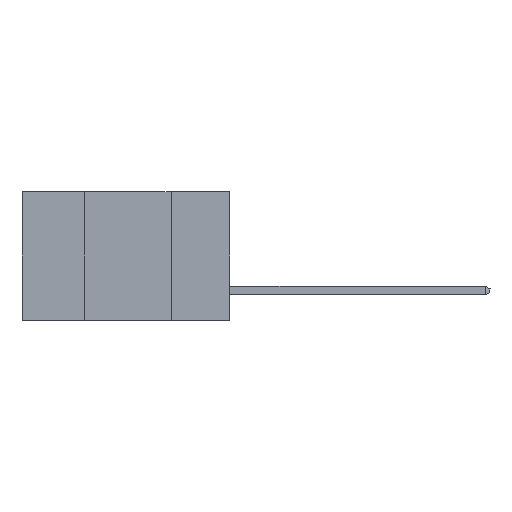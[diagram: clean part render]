
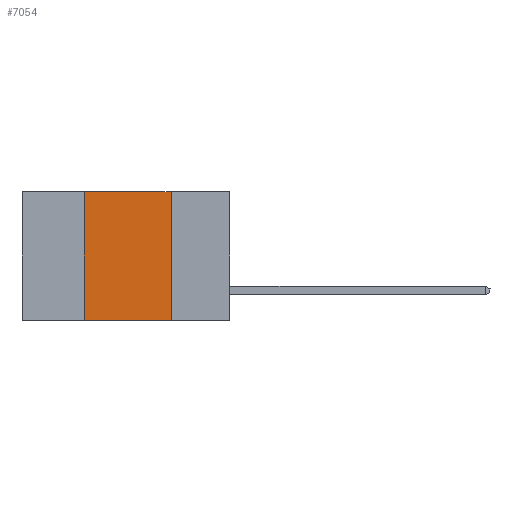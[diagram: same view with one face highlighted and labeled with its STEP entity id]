
A CAD part, left-side view. The second image highlights one B-rep face of the part: STEP entity #7054.
In plain terms, the highlighted planar face has unit normal (-1, 0, 0).
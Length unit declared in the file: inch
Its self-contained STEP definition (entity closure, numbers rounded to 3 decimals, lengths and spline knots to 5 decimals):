
#349 = CARTESIAN_POINT ( 'NONE',  ( 0., 0.6, 0. ) ) ;
#398 = VECTOR ( 'NONE', #7942, 39.37008 ) ;
#472 = CARTESIAN_POINT ( 'NONE',  ( 0., 0.17, 0. ) ) ;
#511 = CARTESIAN_POINT ( 'NONE',  ( 0., 0.42, 0. ) ) ;
#858 = VECTOR ( 'NONE', #1346, 39.37008 ) ;
#1288 = CARTESIAN_POINT ( 'NONE',  ( 0., 0.17, -0.37 ) ) ;
#1346 = DIRECTION ( 'NONE',  ( 0., -1., 0. ) ) ;
#2298 = CARTESIAN_POINT ( 'NONE',  ( 0., 0.6, -0.37 ) ) ;
#2916 = EDGE_CURVE ( 'NONE', #11354, #6321, #6227, .T. ) ;
#3241 = LINE ( 'NONE', #349, #7629 ) ;
#3718 = DIRECTION ( 'NONE',  ( 0., 0., -1. ) ) ;
#3831 = VECTOR ( 'NONE', #9701, 39.37008 ) ;
#4133 = LINE ( 'NONE', #8748, #398 ) ;
#4154 = EDGE_CURVE ( 'NONE', #11354, #4157, #5751, .T. ) ;
#4157 = VERTEX_POINT ( 'NONE', #511 ) ;
#5074 = EDGE_CURVE ( 'NONE', #4157, #11712, #3241, .T. ) ;
#5171 = ORIENTED_EDGE ( 'NONE', *, *, #12190, .F. ) ;
#5327 = FACE_OUTER_BOUND ( 'NONE', #8005, .T. ) ;
#5512 = DIRECTION ( 'NONE',  ( 1., 0., 0. ) ) ;
#5751 = LINE ( 'NONE', #5878, #3831 ) ;
#5878 = CARTESIAN_POINT ( 'NONE',  ( 0., 0.42, -0.37 ) ) ;
#6039 = DIRECTION ( 'NONE',  ( 0., -1., 0. ) ) ;
#6227 = LINE ( 'NONE', #2298, #858 ) ;
#6321 = VERTEX_POINT ( 'NONE', #1288 ) ;
#7054 = ADVANCED_FACE ( 'NONE', ( #5327 ), #10348, .F. ) ;
#7629 = VECTOR ( 'NONE', #6039, 39.37008 ) ;
#7942 = DIRECTION ( 'NONE',  ( 0., 0., -1. ) ) ;
#8005 = EDGE_LOOP ( 'NONE', ( #5171, #10613, #8913, #9086 ) ) ;
#8476 = CARTESIAN_POINT ( 'NONE',  ( 0., 0.42, -0.37 ) ) ;
#8748 = CARTESIAN_POINT ( 'NONE',  ( 0., 0.17, -0.37 ) ) ;
#8878 = AXIS2_PLACEMENT_3D ( 'NONE', #9462, #5512, #3718 ) ;
#8913 = ORIENTED_EDGE ( 'NONE', *, *, #4154, .F. ) ;
#9086 = ORIENTED_EDGE ( 'NONE', *, *, #2916, .T. ) ;
#9462 = CARTESIAN_POINT ( 'NONE',  ( 0., 0.6, 0. ) ) ;
#9701 = DIRECTION ( 'NONE',  ( 0., 0., 1. ) ) ;
#10348 = PLANE ( 'NONE',  #8878 ) ;
#10613 = ORIENTED_EDGE ( 'NONE', *, *, #5074, .F. ) ;
#11354 = VERTEX_POINT ( 'NONE', #8476 ) ;
#11712 = VERTEX_POINT ( 'NONE', #472 ) ;
#12190 = EDGE_CURVE ( 'NONE', #11712, #6321, #4133, .T. ) ;
